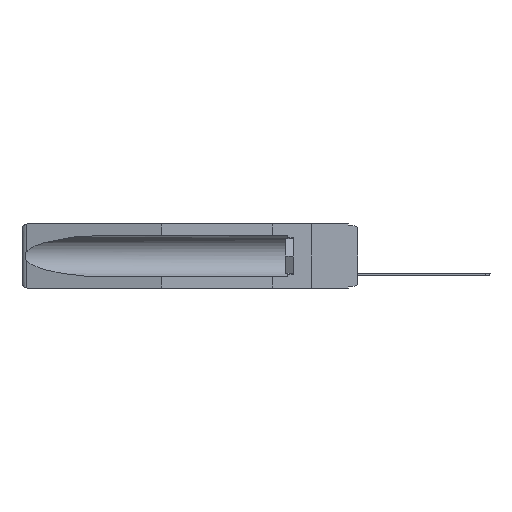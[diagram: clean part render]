
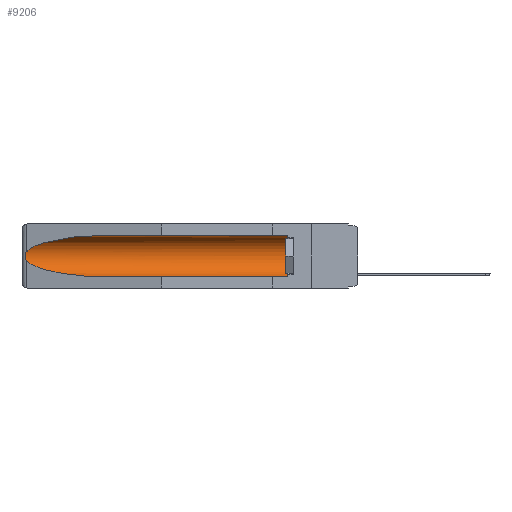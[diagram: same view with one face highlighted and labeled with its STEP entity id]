
A CAD part, left-side view. The second image highlights one B-rep face of the part: STEP entity #9206.
In plain terms, the highlighted cylindrical face has radius 2.857 mm (diameter 5.715 mm), a partial arc.
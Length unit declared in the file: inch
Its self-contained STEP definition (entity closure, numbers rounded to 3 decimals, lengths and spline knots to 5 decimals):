
#950 = DIRECTION ( 'NONE',  ( 0., 1., 0. ) ) ;
#1060 = CARTESIAN_POINT ( 'NONE',  ( 0.26597, 1.5296, -0.19026 ) ) ;
#1180 = DIRECTION ( 'NONE',  ( 0., 1., 0. ) ) ;
#1662 = CARTESIAN_POINT ( 'NONE',  ( 0.155, 0.126, -0.059 ) ) ;
#1801 = AXIS2_PLACEMENT_3D ( 'NONE', #15541, #25922, #13388 ) ;
#2188 = VERTEX_POINT ( 'NONE', #1662 ) ;
#3482 = B_SPLINE_CURVE_WITH_KNOTS ( 'NONE', 3,
 ( #13358, #9578, #11070, #19558, #7418, #17396, #17270, #19425, #1060, #25620 ),
 .UNSPECIFIED., .F., .F.,
 ( 4, 2, 2, 2, 4 ),
 ( 0., 0.00029, 0.00058, 0.00087, 0.00117 ),
 .UNSPECIFIED. ) ;
#3760 = VERTEX_POINT ( 'NONE', #25268 ) ;
#4041 = EDGE_CURVE ( 'NONE', #24165, #16581, #9173, .T. ) ;
#5593 = VECTOR ( 'NONE', #1180, 39.37008 ) ;
#5644 = CARTESIAN_POINT ( 'NONE',  ( 0.26537, 1.52718, -0.14972 ) ) ;
#5896 = ORIENTED_EDGE ( 'NONE', *, *, #14143, .T. ) ;
#6712 = AXIS2_PLACEMENT_3D ( 'NONE', #16959, #25433, #7094 ) ;
#7094 = DIRECTION ( 'NONE',  ( 0., 0., 1. ) ) ;
#7418 = CARTESIAN_POINT ( 'NONE',  ( 0.2675, 1.53308, -0.16763 ) ) ;
#7516 = CARTESIAN_POINT ( 'NONE',  ( 0.21114, 1.30732, -0.059 ) ) ;
#7757 = VECTOR ( 'NONE', #950, 39.37008 ) ;
#8272 = CARTESIAN_POINT ( 'NONE',  ( 0.21114, 1.30732, -0.284 ) ) ;
#9173 =( BOUNDED_CURVE ( )  B_SPLINE_CURVE ( 3, ( #12188, #12327, #8272, #26604 ),
 .UNSPECIFIED., .F., .F. ) 
 B_SPLINE_CURVE_WITH_KNOTS ( ( 4, 4 ),
 ( 0.1948, 1.5708 ),
 .UNSPECIFIED. ) 
 CURVE ( )  GEOMETRIC_REPRESENTATION_ITEM ( )  RATIONAL_B_SPLINE_CURVE ( ( 1., 0.848, 0.848, 1. ) ) 
 REPRESENTATION_ITEM ( '' )  );
#9206 = ADVANCED_FACE ( 'NONE', ( #11504 ), #11771, .F. ) ;
#9578 = CARTESIAN_POINT ( 'NONE',  ( 0.26597, 1.52961, -0.15275 ) ) ;
#9671 = CARTESIAN_POINT ( 'NONE',  ( 0.25451, 1.48313, -0.09465 ) ) ;
#9695 = EDGE_CURVE ( 'NONE', #13588, #24165, #3482, .T. ) ;
#10310 = ORIENTED_EDGE ( 'NONE', *, *, #26585, .F. ) ;
#10615 = CARTESIAN_POINT ( 'NONE',  ( 0.155, 0.126, -0.284 ) ) ;
#11070 = CARTESIAN_POINT ( 'NONE',  ( 0.26654, 1.53092, -0.15636 ) ) ;
#11195 = EDGE_CURVE ( 'NONE', #22461, #2188, #26090, .T. ) ;
#11471 = CARTESIAN_POINT ( 'NONE',  ( 0.155, -0.30754, -0.059 ) ) ;
#11504 = FACE_OUTER_BOUND ( 'NONE', #15333, .T. ) ;
#11771 = CYLINDRICAL_SURFACE ( 'NONE', #1801, 0.1125 ) ;
#12188 = CARTESIAN_POINT ( 'NONE',  ( 0.26537, 1.52718, -0.19328 ) ) ;
#12327 = CARTESIAN_POINT ( 'NONE',  ( 0.25451, 1.48313, -0.24835 ) ) ;
#13358 = CARTESIAN_POINT ( 'NONE',  ( 0.26537, 1.52718, -0.14972 ) ) ;
#13388 = DIRECTION ( 'NONE',  ( 0., 0., 1. ) ) ;
#13588 = VERTEX_POINT ( 'NONE', #5644 ) ;
#14143 = EDGE_CURVE ( 'NONE', #2188, #3760, #19819, .T. ) ;
#14689 =( BOUNDED_CURVE ( )  B_SPLINE_CURVE ( 3, ( #21548, #7516, #9671, #15747 ),
 .UNSPECIFIED., .F., .F. ) 
 B_SPLINE_CURVE_WITH_KNOTS ( ( 4, 4 ),
 ( 4.71239, 6.08839 ),
 .UNSPECIFIED. ) 
 CURVE ( )  GEOMETRIC_REPRESENTATION_ITEM ( )  RATIONAL_B_SPLINE_CURVE ( ( 1., 0.848, 0.848, 1. ) ) 
 REPRESENTATION_ITEM ( '' )  );
#15333 = EDGE_LOOP ( 'NONE', ( #15896, #16164, #19374, #10310, #21566, #5896 ) ) ;
#15541 = CARTESIAN_POINT ( 'NONE',  ( 0.155, -0.30754, -0.1715 ) ) ;
#15747 = CARTESIAN_POINT ( 'NONE',  ( 0.26537, 1.52718, -0.14972 ) ) ;
#15896 = ORIENTED_EDGE ( 'NONE', *, *, #15935, .T. ) ;
#15935 = EDGE_CURVE ( 'NONE', #3760, #13588, #14689, .T. ) ;
#16164 = ORIENTED_EDGE ( 'NONE', *, *, #9695, .T. ) ;
#16581 = VERTEX_POINT ( 'NONE', #25381 ) ;
#16959 = CARTESIAN_POINT ( 'NONE',  ( 0.155, 0.126, -0.1715 ) ) ;
#17270 = CARTESIAN_POINT ( 'NONE',  ( 0.2673, 1.53269, -0.17917 ) ) ;
#17396 = CARTESIAN_POINT ( 'NONE',  ( 0.2675, 1.53308, -0.17534 ) ) ;
#19374 = ORIENTED_EDGE ( 'NONE', *, *, #4041, .T. ) ;
#19425 = CARTESIAN_POINT ( 'NONE',  ( 0.26655, 1.53094, -0.18657 ) ) ;
#19449 = LINE ( 'NONE', #23358, #7757 ) ;
#19558 = CARTESIAN_POINT ( 'NONE',  ( 0.2673, 1.5327, -0.16383 ) ) ;
#19819 = LINE ( 'NONE', #11471, #5593 ) ;
#21548 = CARTESIAN_POINT ( 'NONE',  ( 0.155, 1.07973, -0.059 ) ) ;
#21566 = ORIENTED_EDGE ( 'NONE', *, *, #11195, .T. ) ;
#22461 = VERTEX_POINT ( 'NONE', #10615 ) ;
#23358 = CARTESIAN_POINT ( 'NONE',  ( 0.155, -0.30754, -0.284 ) ) ;
#24165 = VERTEX_POINT ( 'NONE', #25260 ) ;
#25260 = CARTESIAN_POINT ( 'NONE',  ( 0.26537, 1.52718, -0.19328 ) ) ;
#25268 = CARTESIAN_POINT ( 'NONE',  ( 0.155, 1.07973, -0.059 ) ) ;
#25381 = CARTESIAN_POINT ( 'NONE',  ( 0.155, 1.07973, -0.284 ) ) ;
#25433 = DIRECTION ( 'NONE',  ( 0., -1., 0. ) ) ;
#25620 = CARTESIAN_POINT ( 'NONE',  ( 0.26537, 1.52718, -0.19328 ) ) ;
#25922 = DIRECTION ( 'NONE',  ( 0., 1., 0. ) ) ;
#26090 = CIRCLE ( 'NONE', #6712, 0.1125 ) ;
#26585 = EDGE_CURVE ( 'NONE', #22461, #16581, #19449, .T. ) ;
#26604 = CARTESIAN_POINT ( 'NONE',  ( 0.155, 1.07973, -0.284 ) ) ;
